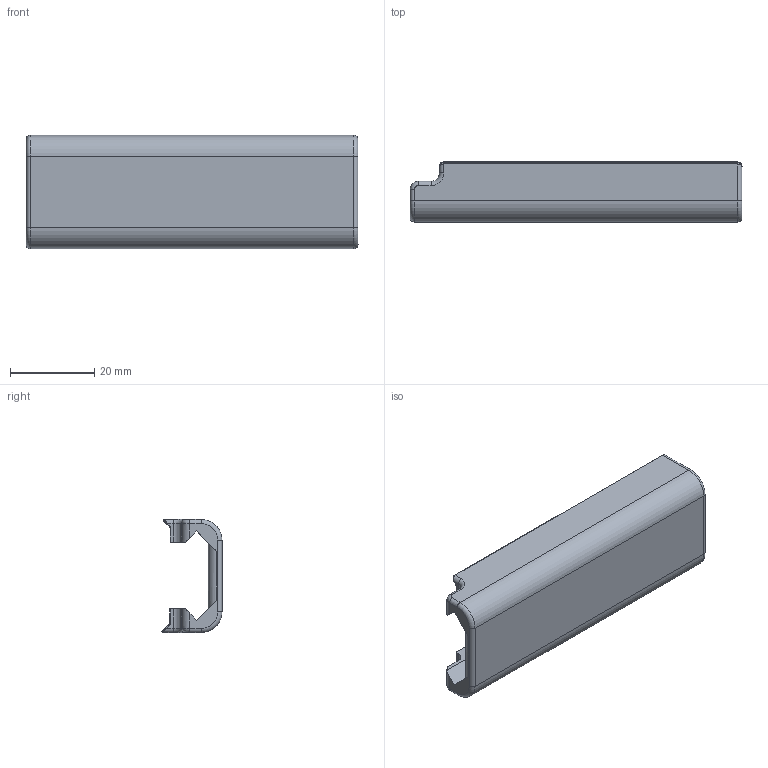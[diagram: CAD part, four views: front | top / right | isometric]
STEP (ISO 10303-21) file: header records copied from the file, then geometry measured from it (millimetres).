
FILE_DESCRIPTION(/* description */ (''),/* implementation_level */ '2;1');
FILE_NAME(/* name */ 'Auto 40L Rail Cover.step',/* time_stamp */ '2021-07-12T09:01:38-06:00',/* author */ (''),/* organization */ (''),/* preprocessor_version */ 'ST-DEVELOPER v18.1',/* originating_system */ 'Autodesk Translation Framework v10.9.0.1377',/* authorisation */ '');
FILE_SCHEMA (('AUTOMOTIVE_DESIGN { 1 0 10303 214 3 1 1 }'));
Length unit declared in the file: millimetre
Products named in the file (1): FNS Release
Bounding box: 78.97 x 14.29 x 26.93 mm (x, y, z)
Volume: 12937.4 mm3; surface area: 8164.4 mm2
Topology: 1 solids, 1 shells, 66 faces, 160 edges, 95 vertices
Faces by surface type: cylinder 28, plane 20, bspline 10, torus 8
Entity records: 2178 total; most frequent: CARTESIAN_POINT 606, DIRECTION 342, ORIENTED_EDGE 314, EDGE_CURVE 157, AXIS2_PLACEMENT_3D 131, VERTEX_POINT 94, LINE 80, VECTOR 80
